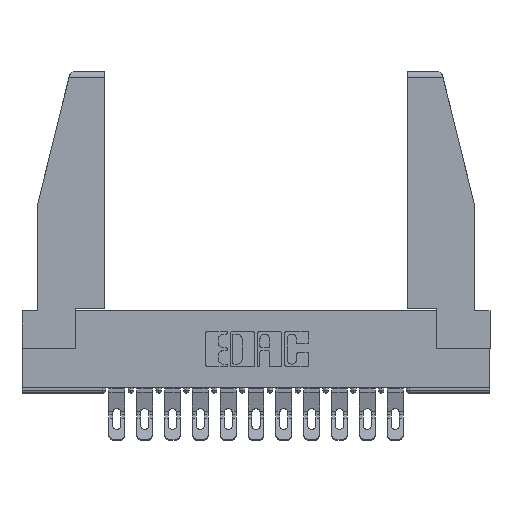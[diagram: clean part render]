
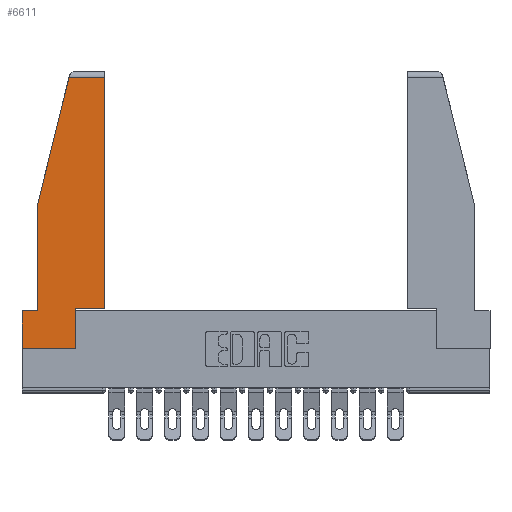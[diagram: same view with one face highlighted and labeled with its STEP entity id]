
A CAD part, top view. The second image highlights one B-rep face of the part: STEP entity #6611.
In plain terms, the highlighted planar face has unit normal (0, 0, 1).
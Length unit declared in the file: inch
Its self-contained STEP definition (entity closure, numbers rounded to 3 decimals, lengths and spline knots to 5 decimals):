
#361 = VECTOR ( 'NONE', #18335, 39.37008 ) ;
#585 = ORIENTED_EDGE ( 'NONE', *, *, #15406, .T. ) ;
#856 = CARTESIAN_POINT ( 'NONE',  ( 0.461, 0.223, 0. ) ) ;
#951 = LINE ( 'NONE', #11237, #9759 ) ;
#1364 = ORIENTED_EDGE ( 'NONE', *, *, #5146, .T. ) ;
#1457 = CARTESIAN_POINT ( 'NONE',  ( 0.086, 0.8, 0. ) ) ;
#1890 = CARTESIAN_POINT ( 'NONE',  ( 0.086, 0.21, 0. ) ) ;
#1984 = VERTEX_POINT ( 'NONE', #8416 ) ;
#2153 = LINE ( 'NONE', #4293, #14123 ) ;
#2221 = CARTESIAN_POINT ( 'NONE',  ( 0.2636, 1.52, 0. ) ) ;
#2383 = CARTESIAN_POINT ( 'NONE',  ( 0.086, 0.8, 0. ) ) ;
#2482 = EDGE_CURVE ( 'NONE', #11393, #9769, #14869, .T. ) ;
#2593 = CARTESIAN_POINT ( 'NONE',  ( 0., 0., 0. ) ) ;
#2915 = EDGE_LOOP ( 'NONE', ( #6373, #15508, #17274, #6460, #13696, #17557, #1364, #585, #5579 ) ) ;
#3448 = EDGE_CURVE ( 'NONE', #9769, #4524, #14606, .T. ) ;
#3490 = DIRECTION ( 'NONE',  ( 0., 1., 0. ) ) ;
#3503 = LINE ( 'NONE', #2383, #361 ) ;
#3789 = EDGE_CURVE ( 'NONE', #17511, #1984, #16395, .T. ) ;
#3815 = CARTESIAN_POINT ( 'NONE',  ( 0.297, 0.223, 0. ) ) ;
#4293 = CARTESIAN_POINT ( 'NONE',  ( 0., 0., 0. ) ) ;
#4486 = DIRECTION ( 'NONE',  ( 1., 0., 0. ) ) ;
#4524 = VERTEX_POINT ( 'NONE', #1457 ) ;
#4832 = EDGE_CURVE ( 'NONE', #4524, #17511, #3503, .T. ) ;
#5146 = EDGE_CURVE ( 'NONE', #6990, #8534, #2153, .T. ) ;
#5579 = ORIENTED_EDGE ( 'NONE', *, *, #15319, .T. ) ;
#5951 = DIRECTION ( 'NONE',  ( -0.239, -0.971, 0. ) ) ;
#5999 = CARTESIAN_POINT ( 'NONE',  ( 0.461, 1.52, 0. ) ) ;
#6373 = ORIENTED_EDGE ( 'NONE', *, *, #6588, .T. ) ;
#6375 = VECTOR ( 'NONE', #3490, 39.37008 ) ;
#6394 = VECTOR ( 'NONE', #15435, 39.37008 ) ;
#6460 = ORIENTED_EDGE ( 'NONE', *, *, #4832, .T. ) ;
#6588 = EDGE_CURVE ( 'NONE', #17649, #11393, #951, .T. ) ;
#6611 = ADVANCED_FACE ( 'NONE', ( #14749 ), #11308, .T. ) ;
#6954 = DIRECTION ( 'NONE',  ( 1., 0., 0. ) ) ;
#6990 = VERTEX_POINT ( 'NONE', #7695 ) ;
#7000 = CARTESIAN_POINT ( 'NONE',  ( 0., 0.21, 0. ) ) ;
#7141 = DIRECTION ( 'NONE',  ( -1., 0., 0. ) ) ;
#7556 = AXIS2_PLACEMENT_3D ( 'NONE', #2593, #15594, #6954 ) ;
#7695 = CARTESIAN_POINT ( 'NONE',  ( 0., 0., 0. ) ) ;
#7756 = LINE ( 'NONE', #3815, #6394 ) ;
#8416 = CARTESIAN_POINT ( 'NONE',  ( 0., 0.21, 0. ) ) ;
#8534 = VERTEX_POINT ( 'NONE', #14173 ) ;
#8677 = LINE ( 'NONE', #9523, #15890 ) ;
#8762 = VECTOR ( 'NONE', #9229, 39.37008 ) ;
#9229 = DIRECTION ( 'NONE',  ( -1., 0., 0. ) ) ;
#9523 = CARTESIAN_POINT ( 'NONE',  ( 0., 0.21, 0. ) ) ;
#9759 = VECTOR ( 'NONE', #12711, 39.37008 ) ;
#9769 = VERTEX_POINT ( 'NONE', #2221 ) ;
#9815 = VECTOR ( 'NONE', #7141, 39.37008 ) ;
#10434 = VERTEX_POINT ( 'NONE', #18101 ) ;
#10930 = CARTESIAN_POINT ( 'NONE',  ( 0.297, 0., 0. ) ) ;
#11237 = CARTESIAN_POINT ( 'NONE',  ( 0.461, 0.223, 0. ) ) ;
#11308 = PLANE ( 'NONE',  #7556 ) ;
#11393 = VERTEX_POINT ( 'NONE', #5999 ) ;
#12119 = VECTOR ( 'NONE', #5951, 39.37008 ) ;
#12711 = DIRECTION ( 'NONE',  ( 0., 1., 0. ) ) ;
#13696 = ORIENTED_EDGE ( 'NONE', *, *, #3789, .T. ) ;
#14123 = VECTOR ( 'NONE', #4486, 39.37008 ) ;
#14173 = CARTESIAN_POINT ( 'NONE',  ( 0.297, 0., 0. ) ) ;
#14562 = EDGE_CURVE ( 'NONE', #1984, #6990, #8677, .T. ) ;
#14606 = LINE ( 'NONE', #15972, #12119 ) ;
#14749 = FACE_OUTER_BOUND ( 'NONE', #2915, .T. ) ;
#14869 = LINE ( 'NONE', #16568, #8762 ) ;
#15319 = EDGE_CURVE ( 'NONE', #10434, #17649, #7756, .T. ) ;
#15406 = EDGE_CURVE ( 'NONE', #8534, #10434, #18644, .T. ) ;
#15435 = DIRECTION ( 'NONE',  ( 1., 0., 0. ) ) ;
#15508 = ORIENTED_EDGE ( 'NONE', *, *, #2482, .T. ) ;
#15594 = DIRECTION ( 'NONE',  ( 0., 0., 1. ) ) ;
#15890 = VECTOR ( 'NONE', #18157, 39.37008 ) ;
#15972 = CARTESIAN_POINT ( 'NONE',  ( 0.271, 1.55, 0. ) ) ;
#16395 = LINE ( 'NONE', #7000, #9815 ) ;
#16568 = CARTESIAN_POINT ( 'NONE',  ( 0., 1.52, 0. ) ) ;
#17274 = ORIENTED_EDGE ( 'NONE', *, *, #3448, .T. ) ;
#17511 = VERTEX_POINT ( 'NONE', #1890 ) ;
#17557 = ORIENTED_EDGE ( 'NONE', *, *, #14562, .T. ) ;
#17649 = VERTEX_POINT ( 'NONE', #856 ) ;
#18101 = CARTESIAN_POINT ( 'NONE',  ( 0.297, 0.223, 0. ) ) ;
#18157 = DIRECTION ( 'NONE',  ( 0., -1., 0. ) ) ;
#18335 = DIRECTION ( 'NONE',  ( 0., -1., 0. ) ) ;
#18644 = LINE ( 'NONE', #10930, #6375 ) ;
